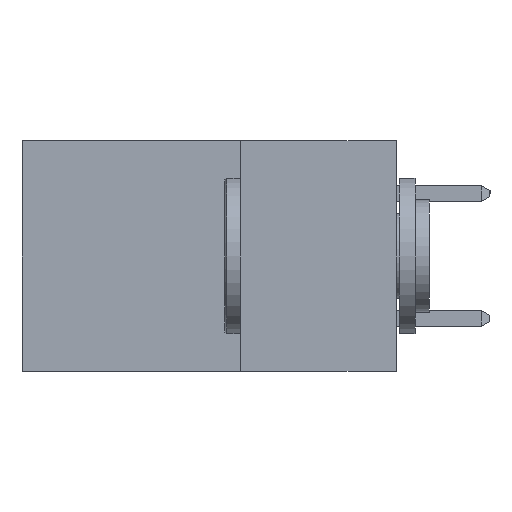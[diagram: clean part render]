
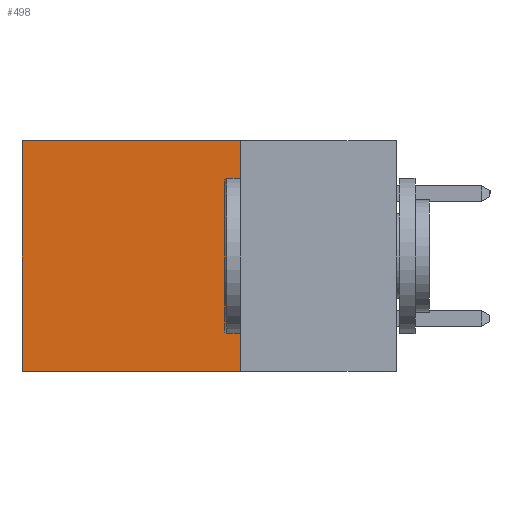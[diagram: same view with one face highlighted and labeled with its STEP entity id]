
A CAD part, left-side view. The second image highlights one B-rep face of the part: STEP entity #498.
In plain terms, the highlighted planar face has unit normal (-1, 0, 0).
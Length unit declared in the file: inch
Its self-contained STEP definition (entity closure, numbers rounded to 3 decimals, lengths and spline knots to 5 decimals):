
#25 = ORIENTED_EDGE ( 'NONE', *, *, #7587, .F. ) ;
#498 = ADVANCED_FACE ( 'NONE', ( #9914 ), #15731, .F. ) ;
#538 = CARTESIAN_POINT ( 'NONE',  ( 0.2615, 0.25, -0.37 ) ) ;
#1308 = ORIENTED_EDGE ( 'NONE', *, *, #7042, .F. ) ;
#1599 = EDGE_CURVE ( 'NONE', #14975, #7899, #1985, .T. ) ;
#1985 = LINE ( 'NONE', #7971, #11287 ) ;
#2076 = DIRECTION ( 'NONE',  ( 0., 0., -1. ) ) ;
#2137 = LINE ( 'NONE', #538, #15316 ) ;
#3549 = DIRECTION ( 'NONE',  ( 0., 0., -1. ) ) ;
#4524 = ORIENTED_EDGE ( 'NONE', *, *, #1599, .T. ) ;
#4630 = EDGE_CURVE ( 'NONE', #11381, #14975, #8945, .T. ) ;
#5476 = LINE ( 'NONE', #11188, #10855 ) ;
#6237 = DIRECTION ( 'NONE',  ( 0., 1., 0. ) ) ;
#7042 = EDGE_CURVE ( 'NONE', #11381, #15154, #2137, .T. ) ;
#7237 = CARTESIAN_POINT ( 'NONE',  ( 0.2615, 0.25, 0. ) ) ;
#7587 = EDGE_CURVE ( 'NONE', #15154, #7899, #5476, .T. ) ;
#7899 = VERTEX_POINT ( 'NONE', #14632 ) ;
#7971 = CARTESIAN_POINT ( 'NONE',  ( 0.2615, 0.6, -0.37 ) ) ;
#8416 = DIRECTION ( 'NONE',  ( 1., 0., 0. ) ) ;
#8945 = LINE ( 'NONE', #17822, #14205 ) ;
#9011 = CARTESIAN_POINT ( 'NONE',  ( 0.2615, 0.25, -0.37 ) ) ;
#9745 = EDGE_LOOP ( 'NONE', ( #4524, #25, #1308, #14070 ) ) ;
#9775 = DIRECTION ( 'NONE',  ( 0., 1., 0. ) ) ;
#9914 = FACE_OUTER_BOUND ( 'NONE', #9745, .T. ) ;
#10190 = CARTESIAN_POINT ( 'NONE',  ( 0.2615, 0.25, -0.37 ) ) ;
#10855 = VECTOR ( 'NONE', #9775, 39.37008 ) ;
#11188 = CARTESIAN_POINT ( 'NONE',  ( 0.2615, 0.25, -0.37 ) ) ;
#11287 = VECTOR ( 'NONE', #2076, 39.37008 ) ;
#11381 = VERTEX_POINT ( 'NONE', #7237 ) ;
#12730 = DIRECTION ( 'NONE',  ( 0., 0., -1. ) ) ;
#14025 = CARTESIAN_POINT ( 'NONE',  ( 0.2615, 0.6, 0. ) ) ;
#14070 = ORIENTED_EDGE ( 'NONE', *, *, #4630, .T. ) ;
#14205 = VECTOR ( 'NONE', #6237, 39.37008 ) ;
#14632 = CARTESIAN_POINT ( 'NONE',  ( 0.2615, 0.6, -0.37 ) ) ;
#14975 = VERTEX_POINT ( 'NONE', #14025 ) ;
#15154 = VERTEX_POINT ( 'NONE', #9011 ) ;
#15316 = VECTOR ( 'NONE', #3549, 39.37008 ) ;
#15411 = AXIS2_PLACEMENT_3D ( 'NONE', #10190, #8416, #12730 ) ;
#15731 = PLANE ( 'NONE',  #15411 ) ;
#17822 = CARTESIAN_POINT ( 'NONE',  ( 0.2615, 0.25, 0. ) ) ;
